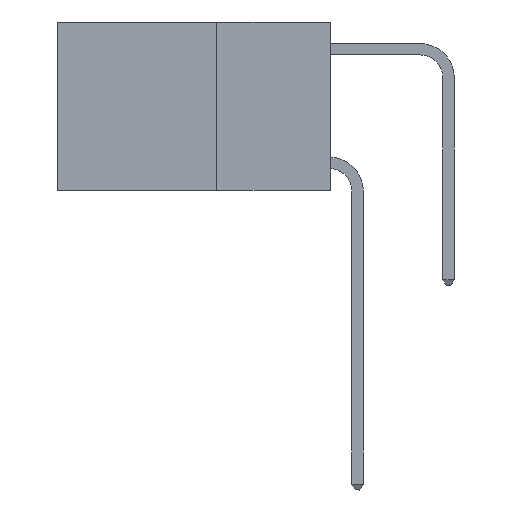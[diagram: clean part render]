
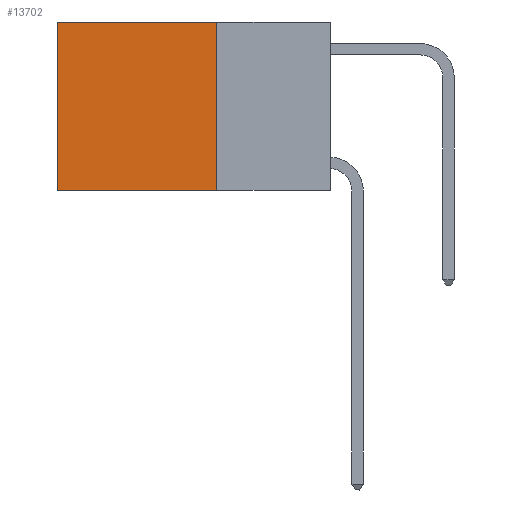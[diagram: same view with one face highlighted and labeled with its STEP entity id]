
A CAD part, left-side view. The second image highlights one B-rep face of the part: STEP entity #13702.
In plain terms, the highlighted planar face has unit normal (-1, 0, 0).
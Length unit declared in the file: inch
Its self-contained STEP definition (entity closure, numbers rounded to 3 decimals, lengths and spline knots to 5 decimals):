
#20 = VERTEX_POINT ( 'NONE', #5245 ) ;
#39 = ORIENTED_EDGE ( 'NONE', *, *, #1674, .T. ) ;
#1116 = CARTESIAN_POINT ( 'NONE',  ( 0.2625, 0.6, 0. ) ) ;
#1535 = LINE ( 'NONE', #5147, #3770 ) ;
#1605 = LINE ( 'NONE', #2633, #12602 ) ;
#1674 = EDGE_CURVE ( 'NONE', #2625, #5985, #6133, .T. ) ;
#1715 = EDGE_CURVE ( 'NONE', #2625, #20, #10972, .T. ) ;
#2056 = ORIENTED_EDGE ( 'NONE', *, *, #1715, .F. ) ;
#2242 = CARTESIAN_POINT ( 'NONE',  ( 0.2625, 0.25, 0. ) ) ;
#2625 = VERTEX_POINT ( 'NONE', #12176 ) ;
#2633 = CARTESIAN_POINT ( 'NONE',  ( 0.2625, 0.25, -0.37 ) ) ;
#3227 = CARTESIAN_POINT ( 'NONE',  ( 0.2625, 0.25, 0. ) ) ;
#3258 = AXIS2_PLACEMENT_3D ( 'NONE', #3227, #5469, #13114 ) ;
#3770 = VECTOR ( 'NONE', #4038, 39.37008 ) ;
#4038 = DIRECTION ( 'NONE',  ( 0., 0., -1. ) ) ;
#4697 = CARTESIAN_POINT ( 'NONE',  ( 0.2625, 0.6, -0.37 ) ) ;
#4999 = DIRECTION ( 'NONE',  ( 0., 0., -1. ) ) ;
#5039 = ORIENTED_EDGE ( 'NONE', *, *, #11692, .F. ) ;
#5147 = CARTESIAN_POINT ( 'NONE',  ( 0.2625, 0.6, 0. ) ) ;
#5245 = CARTESIAN_POINT ( 'NONE',  ( 0.2625, 0.25, -0.37 ) ) ;
#5469 = DIRECTION ( 'NONE',  ( 1., 0., 0. ) ) ;
#5601 = CARTESIAN_POINT ( 'NONE',  ( 0.2625, 0.25, 0. ) ) ;
#5747 = VERTEX_POINT ( 'NONE', #4697 ) ;
#5816 = VECTOR ( 'NONE', #13931, 39.37008 ) ;
#5985 = VERTEX_POINT ( 'NONE', #1116 ) ;
#6133 = LINE ( 'NONE', #2242, #5816 ) ;
#6419 = EDGE_CURVE ( 'NONE', #5985, #5747, #1535, .T. ) ;
#6530 = FACE_OUTER_BOUND ( 'NONE', #8684, .T. ) ;
#8065 = VECTOR ( 'NONE', #4999, 39.37008 ) ;
#8684 = EDGE_LOOP ( 'NONE', ( #12434, #5039, #2056, #39 ) ) ;
#10972 = LINE ( 'NONE', #5601, #8065 ) ;
#11447 = DIRECTION ( 'NONE',  ( 0., 1., 0. ) ) ;
#11692 = EDGE_CURVE ( 'NONE', #20, #5747, #1605, .T. ) ;
#12176 = CARTESIAN_POINT ( 'NONE',  ( 0.2625, 0.25, 0. ) ) ;
#12434 = ORIENTED_EDGE ( 'NONE', *, *, #6419, .T. ) ;
#12602 = VECTOR ( 'NONE', #11447, 39.37008 ) ;
#13114 = DIRECTION ( 'NONE',  ( 0., 0., -1. ) ) ;
#13702 = ADVANCED_FACE ( 'NONE', ( #6530 ), #14130, .F. ) ;
#13931 = DIRECTION ( 'NONE',  ( 0., 1., 0. ) ) ;
#14130 = PLANE ( 'NONE',  #3258 ) ;
